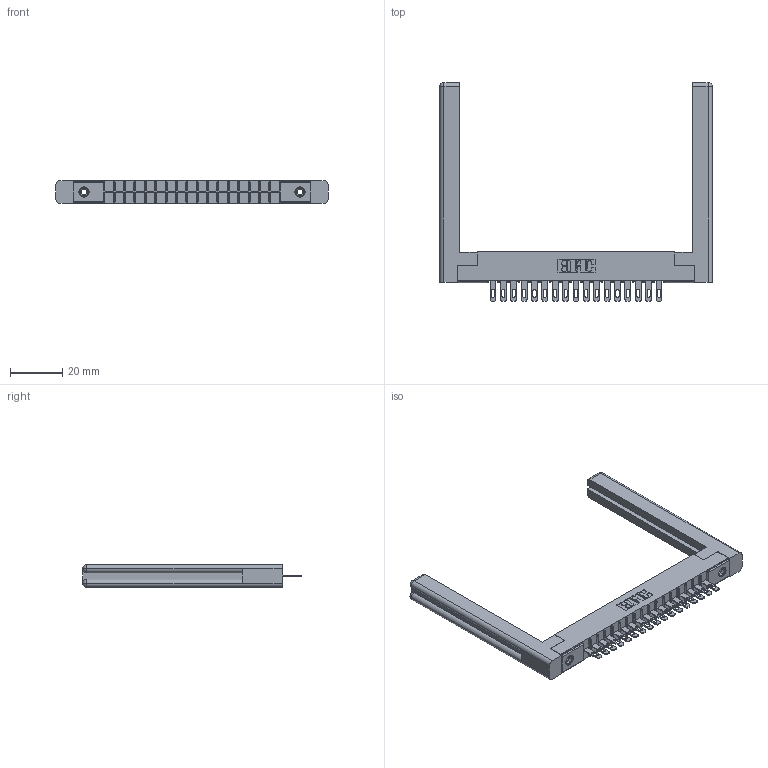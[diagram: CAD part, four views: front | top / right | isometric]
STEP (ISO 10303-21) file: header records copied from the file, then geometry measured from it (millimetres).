
FILE_DESCRIPTION (( 'STEP AP203' ), '1' );
FILE_NAME ('356-017-400-158.STEP', '2020-09-23T12:55:43', ( '' ), ( '' ), 'SwSTEP 2.0', 'SolidWorks 2020', '' );
FILE_SCHEMA (( 'CONFIG_CONTROL_DESIGN' ));
Length unit declared in the file: inch
Products named in the file (5): 306-290-001_100; 306 Part_.156 Dia; 356-017-400-158; 345-250-001_345-250-001-102; 307-220-058
Assembly tree (22 placements, depth 2):
  356-017-400-158
    306 Part_.156 Dia
    306-290-001_100  x17
    345-250-001_345-250-001-102  x2
    307-220-058  x2
Bounding box: 103.99 x 83.52 x 8.71 mm (x, y, z)
Volume: 14786.6 mm3; surface area: 15970.3 mm2
Topology: 22 solids, 22 shells, 1550 faces, 4325 edges, 2778 vertices
Faces by surface type: plane 1002, cylinder 456, sphere 68, cone 12, torus 12
Entity records: 21889 total; most frequent: CARTESIAN_POINT 3681, DIRECTION 3588, ORIENTED_EDGE 3588, EDGE_CURVE 1794, VECTOR 1382, LINE 1382, VERTEX_POINT 1142, AXIS2_PLACEMENT_3D 1103
